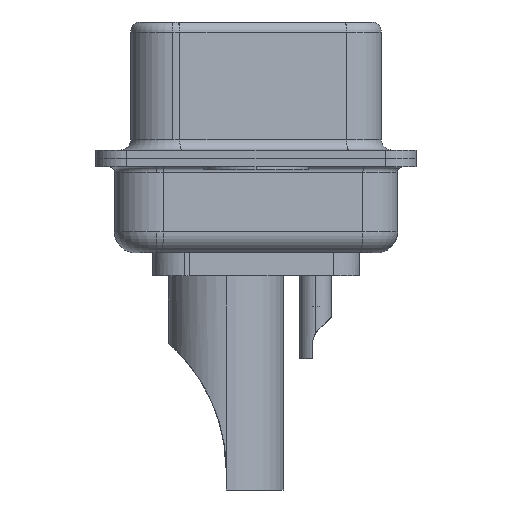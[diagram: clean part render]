
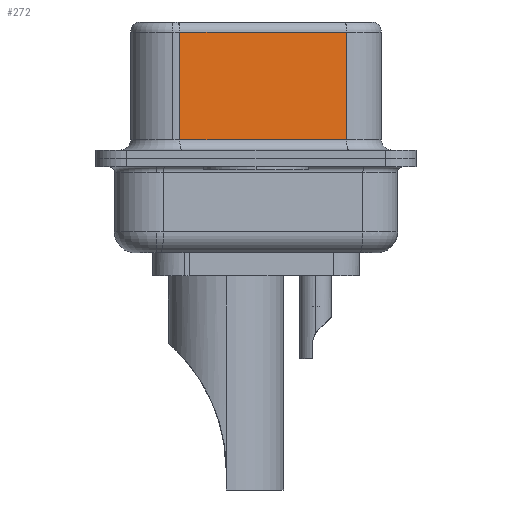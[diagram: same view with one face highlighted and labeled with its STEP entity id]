
A CAD part, left-side view. The second image highlights one B-rep face of the part: STEP entity #272.
In plain terms, the highlighted planar face has unit normal (-0.985, -0.174, 0).
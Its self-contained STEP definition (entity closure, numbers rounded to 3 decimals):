
#272 = ADVANCED_FACE ( 'NONE', ( #1043 ), #14174, .F. ) ;
#1043 = FACE_OUTER_BOUND ( 'NONE', #18923, .T. ) ;
#1139 = CARTESIAN_POINT ( 'NONE',  ( 3.73, 3.628, 6.52 ) ) ;
#1530 = ORIENTED_EDGE ( 'NONE', *, *, #24340, .F. ) ;
#1794 = VECTOR ( 'NONE', #12498, 1000. ) ;
#2171 = AXIS2_PLACEMENT_3D ( 'NONE', #14480, #22214, #14952 ) ;
#2394 = LINE ( 'NONE', #10573, #1794 ) ;
#4033 = VECTOR ( 'NONE', #16404, 1000. ) ;
#5694 = ORIENTED_EDGE ( 'NONE', *, *, #12415, .T. ) ;
#6882 = VERTEX_POINT ( 'NONE', #16444 ) ;
#9775 = DIRECTION ( 'NONE',  ( 0.174, -0.985, 0. ) ) ;
#10254 = VECTOR ( 'NONE', #13348, 1000. ) ;
#10573 = CARTESIAN_POINT ( 'NONE',  ( 5.132, -4.322, 6.52 ) ) ;
#10857 = ORIENTED_EDGE ( 'NONE', *, *, #18315, .T. ) ;
#11496 = VERTEX_POINT ( 'NONE', #18526 ) ;
#12415 = EDGE_CURVE ( 'NONE', #23976, #6882, #14160, .T. ) ;
#12498 = DIRECTION ( 'NONE',  ( 0., 0., -1. ) ) ;
#13089 = CARTESIAN_POINT ( 'NONE',  ( 5.132, -4.322, 6.02 ) ) ;
#13348 = DIRECTION ( 'NONE',  ( -0.174, 0.985, 0. ) ) ;
#14160 = LINE ( 'NONE', #22843, #10254 ) ;
#14174 = PLANE ( 'NONE',  #2171 ) ;
#14480 = CARTESIAN_POINT ( 'NONE',  ( 5.132, -4.322, 6.52 ) ) ;
#14627 = CARTESIAN_POINT ( 'NONE',  ( 3.73, 3.628, 0.9 ) ) ;
#14795 = LINE ( 'NONE', #1139, #4033 ) ;
#14952 = DIRECTION ( 'NONE',  ( -0.174, 0.985, 0. ) ) ;
#15953 = VECTOR ( 'NONE', #9775, 1000. ) ;
#16404 = DIRECTION ( 'NONE',  ( 0., 0., -1. ) ) ;
#16444 = CARTESIAN_POINT ( 'NONE',  ( 3.73, 3.628, 6.02 ) ) ;
#18315 = EDGE_CURVE ( 'NONE', #6882, #19541, #14795, .T. ) ;
#18526 = CARTESIAN_POINT ( 'NONE',  ( 5.132, -4.322, 0.9 ) ) ;
#18687 = EDGE_CURVE ( 'NONE', #19541, #11496, #21635, .T. ) ;
#18923 = EDGE_LOOP ( 'NONE', ( #1530, #5694, #10857, #19207 ) ) ;
#19207 = ORIENTED_EDGE ( 'NONE', *, *, #18687, .T. ) ;
#19541 = VERTEX_POINT ( 'NONE', #14627 ) ;
#21635 = LINE ( 'NONE', #23138, #15953 ) ;
#22214 = DIRECTION ( 'NONE',  ( 0.985, 0.174, 0. ) ) ;
#22843 = CARTESIAN_POINT ( 'NONE',  ( 5.132, -4.322, 6.02 ) ) ;
#23138 = CARTESIAN_POINT ( 'NONE',  ( 5.132, -4.322, 0.9 ) ) ;
#23976 = VERTEX_POINT ( 'NONE', #13089 ) ;
#24340 = EDGE_CURVE ( 'NONE', #23976, #11496, #2394, .T. ) ;
